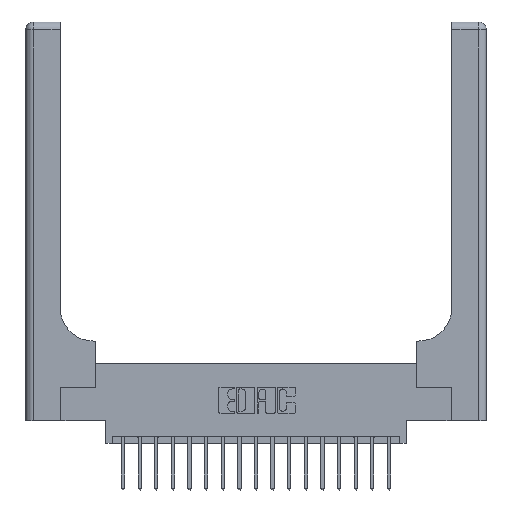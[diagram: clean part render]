
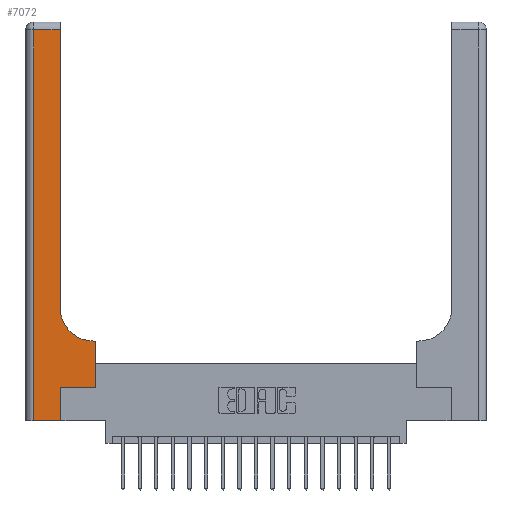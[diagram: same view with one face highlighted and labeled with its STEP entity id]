
A CAD part, top view. The second image highlights one B-rep face of the part: STEP entity #7072.
In plain terms, the highlighted planar face has unit normal (0, 0, 1).
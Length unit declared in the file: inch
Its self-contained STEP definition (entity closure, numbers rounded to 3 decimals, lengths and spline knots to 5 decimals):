
#132 = PLANE ( 'NONE',  #10569 ) ;
#305 = ORIENTED_EDGE ( 'NONE', *, *, #2183, .T. ) ;
#389 = CARTESIAN_POINT ( 'NONE',  ( 0.51, 0.6, 0.37 ) ) ;
#469 = AXIS2_PLACEMENT_3D ( 'NONE', #1963, #12697, #3541 ) ;
#516 = ORIENTED_EDGE ( 'NONE', *, *, #13311, .T. ) ;
#718 = VERTEX_POINT ( 'NONE', #3097 ) ;
#765 = VECTOR ( 'NONE', #3380, 39.37008 ) ;
#1256 = CARTESIAN_POINT ( 'NONE',  ( 0.265, 0., 0.37 ) ) ;
#1676 = DIRECTION ( 'NONE',  ( 0., 0., -1. ) ) ;
#1806 = CARTESIAN_POINT ( 'NONE',  ( 0.528, 0.25, 0.37 ) ) ;
#1937 = VECTOR ( 'NONE', #6498, 39.37008 ) ;
#1963 = CARTESIAN_POINT ( 'NONE',  ( 0.51, 0.85, 0.37 ) ) ;
#2158 = CARTESIAN_POINT ( 'NONE',  ( 0.265, 0.25, 0.37 ) ) ;
#2183 = EDGE_CURVE ( 'NONE', #9733, #18300, #19338, .T. ) ;
#2223 = CARTESIAN_POINT ( 'NONE',  ( 0.26, 0.85, 0.37 ) ) ;
#2391 = VECTOR ( 'NONE', #17150, 39.37008 ) ;
#2933 = EDGE_CURVE ( 'NONE', #18300, #12524, #3613, .T. ) ;
#3097 = CARTESIAN_POINT ( 'NONE',  ( 0.06, 2.94, 0.37 ) ) ;
#3296 = CARTESIAN_POINT ( 'NONE',  ( 0.06, 3., 0.37 ) ) ;
#3376 = ORIENTED_EDGE ( 'NONE', *, *, #13248, .T. ) ;
#3380 = DIRECTION ( 'NONE',  ( 0., 1., 0. ) ) ;
#3541 = DIRECTION ( 'NONE',  ( 1., 0., 0. ) ) ;
#3613 = LINE ( 'NONE', #13943, #11267 ) ;
#5250 = DIRECTION ( 'NONE',  ( 1., 0., 0. ) ) ;
#5741 = CARTESIAN_POINT ( 'NONE',  ( 0.528, 0.6, 0.37 ) ) ;
#6077 = LINE ( 'NONE', #12542, #1937 ) ;
#6217 = LINE ( 'NONE', #3296, #17844 ) ;
#6412 = DIRECTION ( 'NONE',  ( 0., -1., 0. ) ) ;
#6498 = DIRECTION ( 'NONE',  ( -1., 0., 0. ) ) ;
#6826 = FACE_OUTER_BOUND ( 'NONE', #18921, .T. ) ;
#6993 = VERTEX_POINT ( 'NONE', #15157 ) ;
#7072 = ADVANCED_FACE ( 'NONE', ( #6826 ), #132, .F. ) ;
#7122 = ORIENTED_EDGE ( 'NONE', *, *, #7150, .T. ) ;
#7150 = EDGE_CURVE ( 'NONE', #6993, #8235, #8964, .T. ) ;
#7241 = VERTEX_POINT ( 'NONE', #17294 ) ;
#7370 = DIRECTION ( 'NONE',  ( 0., 1., 0. ) ) ;
#7680 = ORIENTED_EDGE ( 'NONE', *, *, #2933, .T. ) ;
#7954 = CARTESIAN_POINT ( 'NONE',  ( 0.26, 2.94, 0.37 ) ) ;
#8235 = VERTEX_POINT ( 'NONE', #5741 ) ;
#8964 = LINE ( 'NONE', #1806, #765 ) ;
#9733 = VERTEX_POINT ( 'NONE', #389 ) ;
#10186 = ORIENTED_EDGE ( 'NONE', *, *, #17514, .T. ) ;
#10569 = AXIS2_PLACEMENT_3D ( 'NONE', #12274, #1676, #12407 ) ;
#10900 = DIRECTION ( 'NONE',  ( 0., 1., 0. ) ) ;
#10938 = CARTESIAN_POINT ( 'NONE',  ( 0.26, 0.6, 0.37 ) ) ;
#11267 = VECTOR ( 'NONE', #10900, 39.37008 ) ;
#11602 = ORIENTED_EDGE ( 'NONE', *, *, #18476, .T. ) ;
#12123 = VECTOR ( 'NONE', #19065, 39.37008 ) ;
#12274 = CARTESIAN_POINT ( 'NONE',  ( 0., 3., 0.37 ) ) ;
#12288 = VERTEX_POINT ( 'NONE', #1256 ) ;
#12407 = DIRECTION ( 'NONE',  ( -1., 0., 0. ) ) ;
#12511 = EDGE_CURVE ( 'NONE', #718, #7241, #6217, .T. ) ;
#12524 = VERTEX_POINT ( 'NONE', #7954 ) ;
#12542 = CARTESIAN_POINT ( 'NONE',  ( 0., 2.94, 0.37 ) ) ;
#12593 = VECTOR ( 'NONE', #7370, 39.37008 ) ;
#12697 = DIRECTION ( 'NONE',  ( 0., 0., -1. ) ) ;
#12946 = CARTESIAN_POINT ( 'NONE',  ( 0., 0., 0.37 ) ) ;
#13053 = LINE ( 'NONE', #14904, #12593 ) ;
#13072 = LINE ( 'NONE', #2158, #17578 ) ;
#13248 = EDGE_CURVE ( 'NONE', #17914, #6993, #13072, .T. ) ;
#13311 = EDGE_CURVE ( 'NONE', #7241, #12288, #16634, .T. ) ;
#13943 = CARTESIAN_POINT ( 'NONE',  ( 0.26, 3., 0.37 ) ) ;
#14904 = CARTESIAN_POINT ( 'NONE',  ( 0.265, 0., 0.37 ) ) ;
#15157 = CARTESIAN_POINT ( 'NONE',  ( 0.528, 0.25, 0.37 ) ) ;
#15230 = ORIENTED_EDGE ( 'NONE', *, *, #12511, .T. ) ;
#16010 = LINE ( 'NONE', #10938, #2391 ) ;
#16469 = CARTESIAN_POINT ( 'NONE',  ( 0.265, 0.25, 0.37 ) ) ;
#16634 = LINE ( 'NONE', #12946, #12123 ) ;
#17055 = EDGE_CURVE ( 'NONE', #12524, #718, #6077, .T. ) ;
#17150 = DIRECTION ( 'NONE',  ( -1., 0., 0. ) ) ;
#17294 = CARTESIAN_POINT ( 'NONE',  ( 0.06, 0., 0.37 ) ) ;
#17514 = EDGE_CURVE ( 'NONE', #8235, #9733, #16010, .T. ) ;
#17578 = VECTOR ( 'NONE', #5250, 39.37008 ) ;
#17844 = VECTOR ( 'NONE', #6412, 39.37008 ) ;
#17914 = VERTEX_POINT ( 'NONE', #16469 ) ;
#18300 = VERTEX_POINT ( 'NONE', #2223 ) ;
#18476 = EDGE_CURVE ( 'NONE', #12288, #17914, #13053, .T. ) ;
#18921 = EDGE_LOOP ( 'NONE', ( #7680, #19155, #15230, #516, #11602, #3376, #7122, #10186, #305 ) ) ;
#19065 = DIRECTION ( 'NONE',  ( 1., 0., 0. ) ) ;
#19155 = ORIENTED_EDGE ( 'NONE', *, *, #17055, .T. ) ;
#19338 = CIRCLE ( 'NONE', #469, 0.25 ) ;
